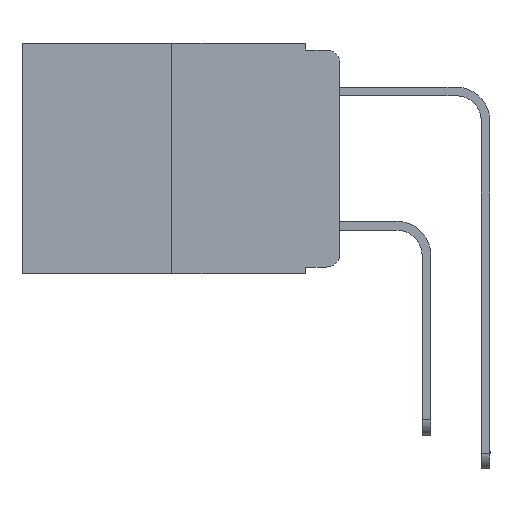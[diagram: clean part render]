
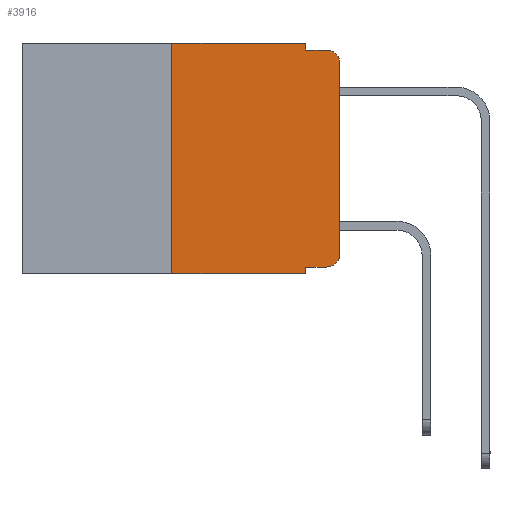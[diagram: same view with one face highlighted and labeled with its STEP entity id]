
A CAD part, left-side view. The second image highlights one B-rep face of the part: STEP entity #3916.
In plain terms, the highlighted planar face has unit normal (-1, 0, 0).
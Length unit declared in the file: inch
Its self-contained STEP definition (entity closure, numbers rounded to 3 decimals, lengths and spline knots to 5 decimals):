
#372 = AXIS2_PLACEMENT_3D ( 'NONE', #1869, #4326, #3215 ) ;
#393 = CARTESIAN_POINT ( 'NONE',  ( 0., 0.02, -0.333 ) ) ;
#460 = VERTEX_POINT ( 'NONE', #393 ) ;
#827 = CARTESIAN_POINT ( 'NONE',  ( 0., 0.051, -0.01 ) ) ;
#1079 = CARTESIAN_POINT ( 'NONE',  ( 0., 0.02, -0.313 ) ) ;
#1167 = EDGE_CURVE ( 'NONE', #3812, #10006, #2653, .T. ) ;
#1181 = DIRECTION ( 'NONE',  ( 0., -1., 0. ) ) ;
#1557 = DIRECTION ( 'NONE',  ( 0., -1., 0. ) ) ;
#1573 = PLANE ( 'NONE',  #3513 ) ;
#1838 = ORIENTED_EDGE ( 'NONE', *, *, #5541, .T. ) ;
#1869 = CARTESIAN_POINT ( 'NONE',  ( 0., 0.02, -0.03 ) ) ;
#2455 = ORIENTED_EDGE ( 'NONE', *, *, #9532, .F. ) ;
#2653 = CIRCLE ( 'NONE', #372, 0.02 ) ;
#2704 = CARTESIAN_POINT ( 'NONE',  ( 0., 0.051, 0. ) ) ;
#2779 = CARTESIAN_POINT ( 'NONE',  ( 0., 0.473, 0. ) ) ;
#3215 = DIRECTION ( 'NONE',  ( 0., 0., -1. ) ) ;
#3358 = CARTESIAN_POINT ( 'NONE',  ( 0., 0.25, 0. ) ) ;
#3434 = CARTESIAN_POINT ( 'NONE',  ( 0., 0.25, 0. ) ) ;
#3513 = AXIS2_PLACEMENT_3D ( 'NONE', #8070, #8208, #9295 ) ;
#3668 = EDGE_CURVE ( 'NONE', #9721, #10006, #10599, .T. ) ;
#3812 = VERTEX_POINT ( 'NONE', #13096 ) ;
#3818 = CARTESIAN_POINT ( 'NONE',  ( 0., 0.02, -0.01 ) ) ;
#3905 = DIRECTION ( 'NONE',  ( 0., 0., -1. ) ) ;
#3916 = ADVANCED_FACE ( 'NONE', ( #11332 ), #1573, .F. ) ;
#3924 = LINE ( 'NONE', #11300, #10205 ) ;
#4104 = CARTESIAN_POINT ( 'NONE',  ( 0., 0.051, -0.01 ) ) ;
#4122 = DIRECTION ( 'NONE',  ( 0., -1., 0. ) ) ;
#4326 = DIRECTION ( 'NONE',  ( -1., 0., 0. ) ) ;
#4403 = EDGE_CURVE ( 'NONE', #5073, #5683, #4864, .T. ) ;
#4425 = EDGE_CURVE ( 'NONE', #9654, #9522, #11449, .T. ) ;
#4531 = EDGE_CURVE ( 'NONE', #7489, #3812, #6212, .T. ) ;
#4864 = LINE ( 'NONE', #2779, #6226 ) ;
#4895 = CARTESIAN_POINT ( 'NONE',  ( 0., 0.051, -0.343 ) ) ;
#5073 = VERTEX_POINT ( 'NONE', #3434 ) ;
#5097 = CARTESIAN_POINT ( 'NONE',  ( 0., 0.051, -0.333 ) ) ;
#5149 = DIRECTION ( 'NONE',  ( 0., 0., 1. ) ) ;
#5541 = EDGE_CURVE ( 'NONE', #460, #7489, #12346, .T. ) ;
#5683 = VERTEX_POINT ( 'NONE', #7988 ) ;
#6207 = ORIENTED_EDGE ( 'NONE', *, *, #4425, .F. ) ;
#6212 = LINE ( 'NONE', #7278, #9636 ) ;
#6226 = VECTOR ( 'NONE', #1557, 39.37008 ) ;
#6261 = AXIS2_PLACEMENT_3D ( 'NONE', #1079, #12798, #6651 ) ;
#6502 = EDGE_CURVE ( 'NONE', #9654, #460, #6544, .T. ) ;
#6544 = LINE ( 'NONE', #10869, #13266 ) ;
#6651 = DIRECTION ( 'NONE',  ( 0., 0., -1. ) ) ;
#6997 = DIRECTION ( 'NONE',  ( 0., 0., -1. ) ) ;
#7103 = VERTEX_POINT ( 'NONE', #10066 ) ;
#7278 = CARTESIAN_POINT ( 'NONE',  ( 0., 0., 0. ) ) ;
#7324 = ORIENTED_EDGE ( 'NONE', *, *, #12769, .F. ) ;
#7489 = VERTEX_POINT ( 'NONE', #12226 ) ;
#7988 = CARTESIAN_POINT ( 'NONE',  ( 0., 0.051, 0. ) ) ;
#8070 = CARTESIAN_POINT ( 'NONE',  ( 0., 0.473, 0. ) ) ;
#8208 = DIRECTION ( 'NONE',  ( 1., 0., 0. ) ) ;
#8399 = ORIENTED_EDGE ( 'NONE', *, *, #3668, .F. ) ;
#9091 = CARTESIAN_POINT ( 'NONE',  ( 0., 0.051, 0. ) ) ;
#9295 = DIRECTION ( 'NONE',  ( 0., 0., -1. ) ) ;
#9457 = ORIENTED_EDGE ( 'NONE', *, *, #4531, .T. ) ;
#9522 = VERTEX_POINT ( 'NONE', #4895 ) ;
#9532 = EDGE_CURVE ( 'NONE', #5683, #9721, #12320, .T. ) ;
#9636 = VECTOR ( 'NONE', #5149, 39.37008 ) ;
#9654 = VERTEX_POINT ( 'NONE', #5097 ) ;
#9694 = ORIENTED_EDGE ( 'NONE', *, *, #13725, .T. ) ;
#9721 = VERTEX_POINT ( 'NONE', #4104 ) ;
#9739 = LINE ( 'NONE', #3358, #9742 ) ;
#9742 = VECTOR ( 'NONE', #10981, 39.37008 ) ;
#9861 = VECTOR ( 'NONE', #6997, 39.37008 ) ;
#9876 = ORIENTED_EDGE ( 'NONE', *, *, #4403, .F. ) ;
#9926 = VECTOR ( 'NONE', #3905, 39.37008 ) ;
#10006 = VERTEX_POINT ( 'NONE', #3818 ) ;
#10066 = CARTESIAN_POINT ( 'NONE',  ( 0., 0.25, -0.343 ) ) ;
#10205 = VECTOR ( 'NONE', #11497, 39.37008 ) ;
#10327 = VECTOR ( 'NONE', #4122, 39.37008 ) ;
#10599 = LINE ( 'NONE', #827, #10327 ) ;
#10869 = CARTESIAN_POINT ( 'NONE',  ( 0., 0.051, -0.333 ) ) ;
#10981 = DIRECTION ( 'NONE',  ( 0., 0., 1. ) ) ;
#11300 = CARTESIAN_POINT ( 'NONE',  ( 0., 0.473, -0.343 ) ) ;
#11332 = FACE_OUTER_BOUND ( 'NONE', #13518, .T. ) ;
#11449 = LINE ( 'NONE', #2704, #9861 ) ;
#11497 = DIRECTION ( 'NONE',  ( 0., -1., 0. ) ) ;
#12226 = CARTESIAN_POINT ( 'NONE',  ( 0., 0., -0.313 ) ) ;
#12320 = LINE ( 'NONE', #9091, #9926 ) ;
#12346 = CIRCLE ( 'NONE', #6261, 0.02 ) ;
#12480 = ORIENTED_EDGE ( 'NONE', *, *, #6502, .T. ) ;
#12769 = EDGE_CURVE ( 'NONE', #7103, #5073, #9739, .T. ) ;
#12798 = DIRECTION ( 'NONE',  ( -1., 0., 0. ) ) ;
#13096 = CARTESIAN_POINT ( 'NONE',  ( 0., 0., -0.03 ) ) ;
#13266 = VECTOR ( 'NONE', #1181, 39.37008 ) ;
#13518 = EDGE_LOOP ( 'NONE', ( #9457, #13731, #8399, #2455, #9876, #7324, #9694, #6207, #12480, #1838 ) ) ;
#13725 = EDGE_CURVE ( 'NONE', #7103, #9522, #3924, .T. ) ;
#13731 = ORIENTED_EDGE ( 'NONE', *, *, #1167, .T. ) ;
